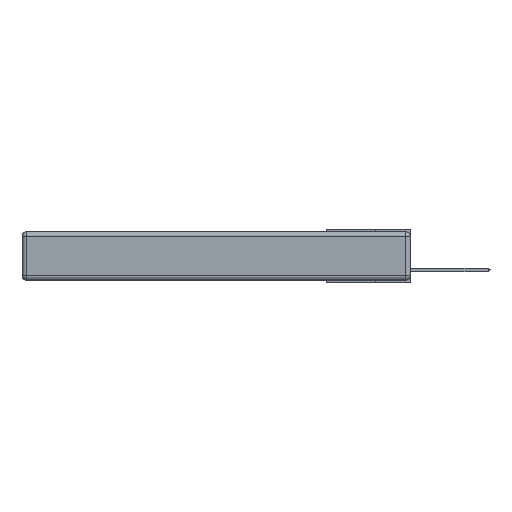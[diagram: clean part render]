
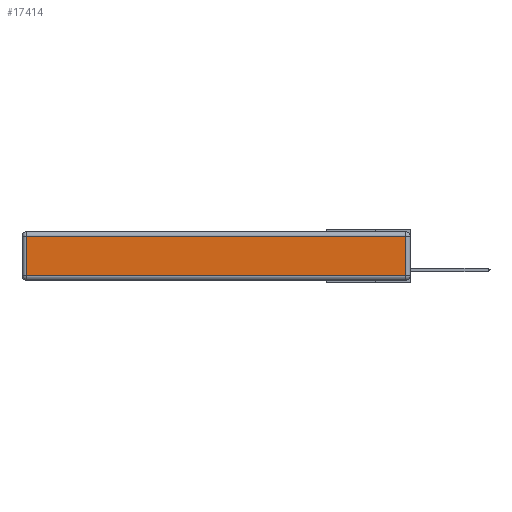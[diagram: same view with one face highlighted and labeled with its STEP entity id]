
A CAD part, left-side view. The second image highlights one B-rep face of the part: STEP entity #17414.
In plain terms, the highlighted planar face has unit normal (-1, 0, 0).
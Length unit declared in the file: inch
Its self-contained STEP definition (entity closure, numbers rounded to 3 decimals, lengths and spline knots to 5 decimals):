
#381 = DIRECTION ( 'NONE',  ( 0., 1., 0. ) ) ;
#1267 = LINE ( 'NONE', #4843, #2160 ) ;
#1525 = VECTOR ( 'NONE', #2883, 39.37008 ) ;
#1764 = CARTESIAN_POINT ( 'NONE',  ( 0., 0., -0.313 ) ) ;
#2160 = VECTOR ( 'NONE', #381, 39.37008 ) ;
#2883 = DIRECTION ( 'NONE',  ( 0., 0., -1. ) ) ;
#2997 = DIRECTION ( 'NONE',  ( 0., 0., 1. ) ) ;
#3875 = CARTESIAN_POINT ( 'NONE',  ( 0., 0.03, -0.343 ) ) ;
#4843 = CARTESIAN_POINT ( 'NONE',  ( 0., 2.75, -0.03 ) ) ;
#4996 = LINE ( 'NONE', #3875, #18677 ) ;
#6113 = DIRECTION ( 'NONE',  ( 0., -1., 0. ) ) ;
#6846 = CARTESIAN_POINT ( 'NONE',  ( 0., 0.03, -0.03 ) ) ;
#6975 = AXIS2_PLACEMENT_3D ( 'NONE', #12512, #13140, #2997 ) ;
#8161 = VERTEX_POINT ( 'NONE', #15573 ) ;
#9937 = EDGE_CURVE ( 'NONE', #17852, #8161, #11179, .T. ) ;
#10554 = ORIENTED_EDGE ( 'NONE', *, *, #9937, .T. ) ;
#10961 = DIRECTION ( 'NONE',  ( 0., 0., 1. ) ) ;
#11156 = FACE_OUTER_BOUND ( 'NONE', #14520, .T. ) ;
#11179 = LINE ( 'NONE', #1764, #13183 ) ;
#12237 = CARTESIAN_POINT ( 'NONE',  ( 0., 2.72, -0.313 ) ) ;
#12512 = CARTESIAN_POINT ( 'NONE',  ( 0., 0., -0.343 ) ) ;
#12722 = PLANE ( 'NONE',  #6975 ) ;
#12927 = CARTESIAN_POINT ( 'NONE',  ( 0., 2.72, -0.343 ) ) ;
#13140 = DIRECTION ( 'NONE',  ( -1., 0., 0. ) ) ;
#13183 = VECTOR ( 'NONE', #6113, 39.37008 ) ;
#14520 = EDGE_LOOP ( 'NONE', ( #10554, #15531, #17963, #15042 ) ) ;
#14790 = EDGE_CURVE ( 'NONE', #8161, #18645, #4996, .T. ) ;
#15042 = ORIENTED_EDGE ( 'NONE', *, *, #16225, .T. ) ;
#15531 = ORIENTED_EDGE ( 'NONE', *, *, #14790, .T. ) ;
#15573 = CARTESIAN_POINT ( 'NONE',  ( 0., 0.03, -0.313 ) ) ;
#15933 = LINE ( 'NONE', #12927, #1525 ) ;
#16225 = EDGE_CURVE ( 'NONE', #17882, #17852, #15933, .T. ) ;
#16650 = EDGE_CURVE ( 'NONE', #18645, #17882, #1267, .T. ) ;
#16860 = CARTESIAN_POINT ( 'NONE',  ( 0., 2.72, -0.03 ) ) ;
#17414 = ADVANCED_FACE ( 'NONE', ( #11156 ), #12722, .T. ) ;
#17852 = VERTEX_POINT ( 'NONE', #12237 ) ;
#17882 = VERTEX_POINT ( 'NONE', #16860 ) ;
#17963 = ORIENTED_EDGE ( 'NONE', *, *, #16650, .T. ) ;
#18645 = VERTEX_POINT ( 'NONE', #6846 ) ;
#18677 = VECTOR ( 'NONE', #10961, 39.37008 ) ;
